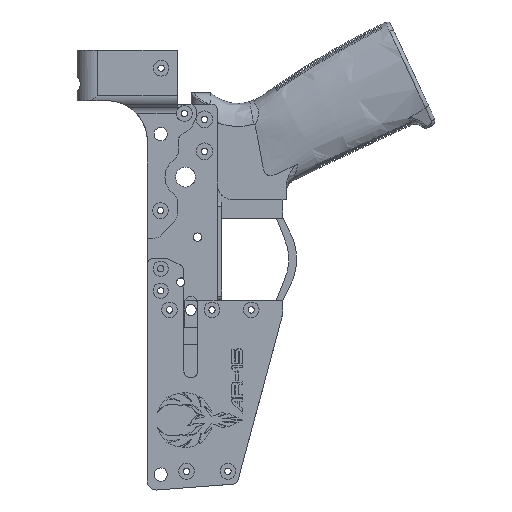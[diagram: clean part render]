
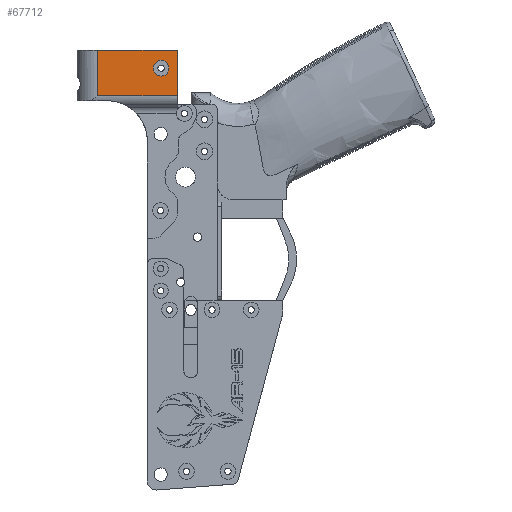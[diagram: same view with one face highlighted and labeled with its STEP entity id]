
A CAD part, left-side view. The second image highlights one B-rep face of the part: STEP entity #67712.
In plain terms, the highlighted planar face has unit normal (-1, 0, 0).
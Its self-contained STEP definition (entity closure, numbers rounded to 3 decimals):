
#513 = DIRECTION ( 'NONE',  ( 0., -1., 0. ) ) ;
#1915 = LINE ( 'NONE', #76711, #69991 ) ;
#6435 = EDGE_LOOP ( 'NONE', ( #29532, #134786, #29001, #12430 ) ) ;
#8387 = EDGE_CURVE ( 'NONE', #30653, #53080, #53241, .T. ) ;
#8544 = LINE ( 'NONE', #83294, #126624 ) ;
#10950 = CARTESIAN_POINT ( 'NONE',  ( -25., -36.779, -288600.29 ) ) ;
#12430 = ORIENTED_EDGE ( 'NONE', *, *, #23514, .T. ) ;
#13083 = EDGE_CURVE ( 'NONE', #53080, #63802, #1915, .T. ) ;
#14448 = AXIS2_PLACEMENT_3D ( 'NONE', #115973, #49619, #74036 ) ;
#14979 = EDGE_CURVE ( 'NONE', #129815, #132558, #36767, .T. ) ;
#23514 = EDGE_CURVE ( 'NONE', #57320, #30653, #8544, .T. ) ;
#29001 = ORIENTED_EDGE ( 'NONE', *, *, #34343, .T. ) ;
#29120 = VECTOR ( 'NONE', #83997, 1000. ) ;
#29141 = AXIS2_PLACEMENT_3D ( 'NONE', #55119, #118004, #97736 ) ;
#29532 = ORIENTED_EDGE ( 'NONE', *, *, #8387, .T. ) ;
#30653 = VERTEX_POINT ( 'NONE', #99453 ) ;
#33983 = DIRECTION ( 'NONE',  ( 0., 0., -1. ) ) ;
#34343 = EDGE_CURVE ( 'NONE', #63802, #57320, #41149, .T. ) ;
#36767 = CIRCLE ( 'NONE', #14448, 3.75 ) ;
#41149 = LINE ( 'NONE', #135533, #102281 ) ;
#47827 = CARTESIAN_POINT ( 'NONE',  ( -25., -30.202, -10.291 ) ) ;
#49619 = DIRECTION ( 'NONE',  ( -1., 0., 0. ) ) ;
#53080 = VERTEX_POINT ( 'NONE', #100897 ) ;
#53241 = LINE ( 'NONE', #137130, #29120 ) ;
#55119 = CARTESIAN_POINT ( 'NONE',  ( -25., -22.502, 2.734 ) ) ;
#57320 = VERTEX_POINT ( 'NONE', #73366 ) ;
#60792 = CARTESIAN_POINT ( 'NONE',  ( -25., -22.502, 6.484 ) ) ;
#62804 = DIRECTION ( 'NONE',  ( 0., 0., 1. ) ) ;
#63802 = VERTEX_POINT ( 'NONE', #47827 ) ;
#64059 = FACE_BOUND ( 'NONE', #107388, .T. ) ;
#67712 = ADVANCED_FACE ( 'NONE', ( #64059, #119924 ), #130421, .F. ) ;
#69991 = VECTOR ( 'NONE', #513, 1000. ) ;
#72127 = DIRECTION ( 'NONE',  ( 0., 1., 0. ) ) ;
#73366 = CARTESIAN_POINT ( 'NONE',  ( -25., -30.202, 11.224 ) ) ;
#73506 = EDGE_CURVE ( 'NONE', #132558, #129815, #127314, .T. ) ;
#74036 = DIRECTION ( 'NONE',  ( 0., 0., 1. ) ) ;
#76711 = CARTESIAN_POINT ( 'NONE',  ( -25., -36.779, -10.291 ) ) ;
#77744 = AXIS2_PLACEMENT_3D ( 'NONE', #10950, #129747, #33983 ) ;
#83294 = CARTESIAN_POINT ( 'NONE',  ( -25., -36.779, 11.224 ) ) ;
#83997 = DIRECTION ( 'NONE',  ( 0., 0., -1. ) ) ;
#92061 = CARTESIAN_POINT ( 'NONE',  ( -25., -22.502, -1.016 ) ) ;
#97736 = DIRECTION ( 'NONE',  ( 0., 0., 1. ) ) ;
#99453 = CARTESIAN_POINT ( 'NONE',  ( -25., 7.678, 11.224 ) ) ;
#100897 = CARTESIAN_POINT ( 'NONE',  ( -25., 7.678, -10.291 ) ) ;
#102281 = VECTOR ( 'NONE', #62804, 1000. ) ;
#107388 = EDGE_LOOP ( 'NONE', ( #117167, #121193 ) ) ;
#115973 = CARTESIAN_POINT ( 'NONE',  ( -25., -22.502, 2.734 ) ) ;
#117167 = ORIENTED_EDGE ( 'NONE', *, *, #14979, .F. ) ;
#118004 = DIRECTION ( 'NONE',  ( -1., 0., 0. ) ) ;
#119924 = FACE_OUTER_BOUND ( 'NONE', #6435, .T. ) ;
#121193 = ORIENTED_EDGE ( 'NONE', *, *, #73506, .F. ) ;
#126624 = VECTOR ( 'NONE', #72127, 1000. ) ;
#127314 = CIRCLE ( 'NONE', #29141, 3.75 ) ;
#129747 = DIRECTION ( 'NONE',  ( 1., 0., 0. ) ) ;
#129815 = VERTEX_POINT ( 'NONE', #60792 ) ;
#130421 = PLANE ( 'NONE',  #77744 ) ;
#132558 = VERTEX_POINT ( 'NONE', #92061 ) ;
#134786 = ORIENTED_EDGE ( 'NONE', *, *, #13083, .T. ) ;
#135533 = CARTESIAN_POINT ( 'NONE',  ( -25., -30.202, -14.306 ) ) ;
#137130 = CARTESIAN_POINT ( 'NONE',  ( -25., 7.678, -12.776 ) ) ;
